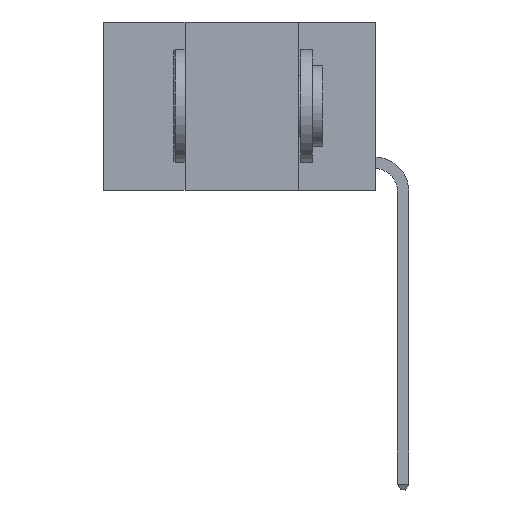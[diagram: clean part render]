
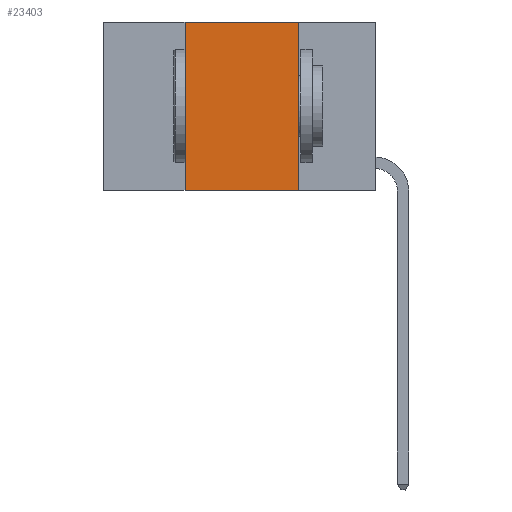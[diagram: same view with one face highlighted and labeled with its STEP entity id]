
A CAD part, left-side view. The second image highlights one B-rep face of the part: STEP entity #23403.
In plain terms, the highlighted planar face has unit normal (-1, 0, 0).
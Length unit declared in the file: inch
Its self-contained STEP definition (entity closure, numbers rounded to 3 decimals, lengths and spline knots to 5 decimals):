
#197 = EDGE_CURVE ( 'NONE', #13224, #14160, #22277, .T. ) ;
#429 = CARTESIAN_POINT ( 'NONE',  ( 0., 0.6, 0. ) ) ;
#1903 = LINE ( 'NONE', #11946, #16625 ) ;
#2488 = DIRECTION ( 'NONE',  ( 0., 0., -1. ) ) ;
#2525 = ORIENTED_EDGE ( 'NONE', *, *, #9954, .T. ) ;
#3485 = CARTESIAN_POINT ( 'NONE',  ( 0., 0.42, 0. ) ) ;
#4401 = EDGE_CURVE ( 'NONE', #14160, #5943, #1903, .T. ) ;
#5943 = VERTEX_POINT ( 'NONE', #10924 ) ;
#6886 = ORIENTED_EDGE ( 'NONE', *, *, #4401, .F. ) ;
#7965 = DIRECTION ( 'NONE',  ( 0., 0., 1. ) ) ;
#8061 = AXIS2_PLACEMENT_3D ( 'NONE', #429, #14483, #2488 ) ;
#8138 = CARTESIAN_POINT ( 'NONE',  ( 0., 0.6, 0. ) ) ;
#8455 = PLANE ( 'NONE',  #8061 ) ;
#8625 = CARTESIAN_POINT ( 'NONE',  ( 0., 0.17, 0. ) ) ;
#8941 = VERTEX_POINT ( 'NONE', #23512 ) ;
#9943 = DIRECTION ( 'NONE',  ( 0., -1., 0. ) ) ;
#9954 = EDGE_CURVE ( 'NONE', #8941, #5943, #11992, .T. ) ;
#10791 = EDGE_LOOP ( 'NONE', ( #6886, #15328, #10804, #2525 ) ) ;
#10804 = ORIENTED_EDGE ( 'NONE', *, *, #15286, .F. ) ;
#10924 = CARTESIAN_POINT ( 'NONE',  ( 0., 0.17, -0.37 ) ) ;
#11946 = CARTESIAN_POINT ( 'NONE',  ( 0., 0.17, 0. ) ) ;
#11992 = LINE ( 'NONE', #19997, #20715 ) ;
#13224 = VERTEX_POINT ( 'NONE', #3485 ) ;
#14160 = VERTEX_POINT ( 'NONE', #8625 ) ;
#14483 = DIRECTION ( 'NONE',  ( 1., 0., 0. ) ) ;
#15286 = EDGE_CURVE ( 'NONE', #8941, #13224, #22999, .T. ) ;
#15328 = ORIENTED_EDGE ( 'NONE', *, *, #197, .F. ) ;
#16625 = VECTOR ( 'NONE', #19887, 39.37008 ) ;
#17596 = VECTOR ( 'NONE', #9943, 39.37008 ) ;
#17697 = VECTOR ( 'NONE', #7965, 39.37008 ) ;
#19887 = DIRECTION ( 'NONE',  ( 0., 0., -1. ) ) ;
#19997 = CARTESIAN_POINT ( 'NONE',  ( 0., 0.6, -0.37 ) ) ;
#20715 = VECTOR ( 'NONE', #24080, 39.37008 ) ;
#22277 = LINE ( 'NONE', #8138, #17596 ) ;
#22514 = FACE_OUTER_BOUND ( 'NONE', #10791, .T. ) ;
#22999 = LINE ( 'NONE', #23839, #17697 ) ;
#23403 = ADVANCED_FACE ( 'NONE', ( #22514 ), #8455, .F. ) ;
#23512 = CARTESIAN_POINT ( 'NONE',  ( 0., 0.42, -0.37 ) ) ;
#23839 = CARTESIAN_POINT ( 'NONE',  ( 0., 0.42, 0. ) ) ;
#24080 = DIRECTION ( 'NONE',  ( 0., -1., 0. ) ) ;
